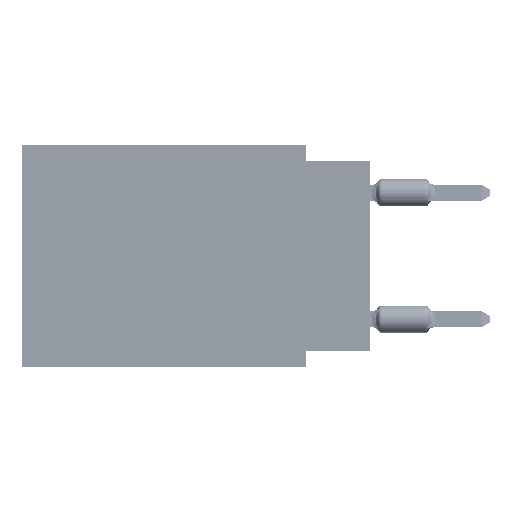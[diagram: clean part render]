
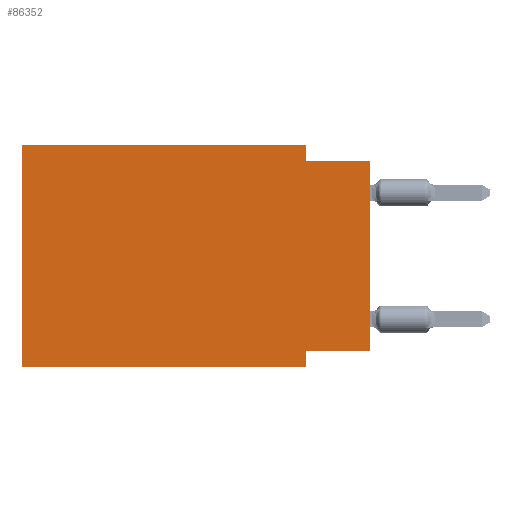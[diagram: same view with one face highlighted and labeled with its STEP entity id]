
A CAD part, left-side view. The second image highlights one B-rep face of the part: STEP entity #86352.
In plain terms, the highlighted planar face has unit normal (-1, 0, 0).
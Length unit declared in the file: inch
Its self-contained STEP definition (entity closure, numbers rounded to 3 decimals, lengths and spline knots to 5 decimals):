
#1003 = ORIENTED_EDGE ( 'NONE', *, *, #39772, .F. ) ;
#2093 = DIRECTION ( 'NONE',  ( 0., 0., -1. ) ) ;
#5446 = DIRECTION ( 'NONE',  ( 0., -1., 0. ) ) ;
#8709 = CARTESIAN_POINT ( 'NONE',  ( 0., 0.1, 0. ) ) ;
#10148 = LINE ( 'NONE', #18905, #48730 ) ;
#13813 = CARTESIAN_POINT ( 'NONE',  ( 0., 0.55, -0.35 ) ) ;
#14261 = LINE ( 'NONE', #49789, #84240 ) ;
#15055 = LINE ( 'NONE', #48445, #47356 ) ;
#15538 = EDGE_CURVE ( 'NONE', #74234, #21049, #10148, .T. ) ;
#16152 = EDGE_CURVE ( 'NONE', #72362, #93234, #98389, .T. ) ;
#17531 = FACE_OUTER_BOUND ( 'NONE', #35085, .T. ) ;
#18905 = CARTESIAN_POINT ( 'NONE',  ( 0., 0., -0.025 ) ) ;
#20301 = VERTEX_POINT ( 'NONE', #31533 ) ;
#21049 = VERTEX_POINT ( 'NONE', #102952 ) ;
#22380 = AXIS2_PLACEMENT_3D ( 'NONE', #33429, #59609, #49814 ) ;
#22952 = CARTESIAN_POINT ( 'NONE',  ( 0., 0.1, -0.325 ) ) ;
#26205 = LINE ( 'NONE', #8709, #44243 ) ;
#26904 = EDGE_CURVE ( 'NONE', #20301, #49916, #27054, .T. ) ;
#27054 = LINE ( 'NONE', #43473, #54297 ) ;
#27501 = ORIENTED_EDGE ( 'NONE', *, *, #15538, .F. ) ;
#27883 = VECTOR ( 'NONE', #5446, 39.37008 ) ;
#27966 = CARTESIAN_POINT ( 'NONE',  ( 0., 0., 0. ) ) ;
#28181 = CARTESIAN_POINT ( 'NONE',  ( 0., 0., -0.325 ) ) ;
#31533 = CARTESIAN_POINT ( 'NONE',  ( 0., 0.55, 0. ) ) ;
#33108 = EDGE_CURVE ( 'NONE', #72362, #20301, #72391, .T. ) ;
#33429 = CARTESIAN_POINT ( 'NONE',  ( 0., 0.55, 0. ) ) ;
#35085 = EDGE_LOOP ( 'NONE', ( #74223, #27501, #106396, #97913, #68588, #54186, #1003, #39846 ) ) ;
#39772 = EDGE_CURVE ( 'NONE', #79829, #93234, #14261, .T. ) ;
#39846 = ORIENTED_EDGE ( 'NONE', *, *, #63535, .F. ) ;
#41630 = PLANE ( 'NONE',  #22380 ) ;
#43473 = CARTESIAN_POINT ( 'NONE',  ( 0., 0.55, 0. ) ) ;
#44243 = VECTOR ( 'NONE', #2093, 39.37008 ) ;
#44535 = VECTOR ( 'NONE', #82196, 39.37008 ) ;
#47356 = VECTOR ( 'NONE', #65923, 39.37008 ) ;
#48445 = CARTESIAN_POINT ( 'NONE',  ( 0., 0., -0.325 ) ) ;
#48730 = VECTOR ( 'NONE', #60441, 39.37008 ) ;
#49789 = CARTESIAN_POINT ( 'NONE',  ( 0., 0.1, -0.35 ) ) ;
#49814 = DIRECTION ( 'NONE',  ( 0., 0., -1. ) ) ;
#49916 = VERTEX_POINT ( 'NONE', #62021 ) ;
#54186 = ORIENTED_EDGE ( 'NONE', *, *, #16152, .T. ) ;
#54297 = VECTOR ( 'NONE', #67006, 39.37008 ) ;
#59609 = DIRECTION ( 'NONE',  ( 1., 0., 0. ) ) ;
#60441 = DIRECTION ( 'NONE',  ( 0., -1., 0. ) ) ;
#62021 = CARTESIAN_POINT ( 'NONE',  ( 0., 0.1, 0. ) ) ;
#63535 = EDGE_CURVE ( 'NONE', #104488, #79829, #15055, .T. ) ;
#65923 = DIRECTION ( 'NONE',  ( 0., 1., 0. ) ) ;
#66745 = DIRECTION ( 'NONE',  ( 0., 0., -1. ) ) ;
#67006 = DIRECTION ( 'NONE',  ( 0., -1., 0. ) ) ;
#68588 = ORIENTED_EDGE ( 'NONE', *, *, #33108, .F. ) ;
#72362 = VERTEX_POINT ( 'NONE', #13813 ) ;
#72391 = LINE ( 'NONE', #90925, #44535 ) ;
#74223 = ORIENTED_EDGE ( 'NONE', *, *, #76300, .T. ) ;
#74234 = VERTEX_POINT ( 'NONE', #105771 ) ;
#76300 = EDGE_CURVE ( 'NONE', #104488, #21049, #103938, .T. ) ;
#79829 = VERTEX_POINT ( 'NONE', #22952 ) ;
#80378 = CARTESIAN_POINT ( 'NONE',  ( 0., 0.55, -0.35 ) ) ;
#82196 = DIRECTION ( 'NONE',  ( 0., 0., 1. ) ) ;
#84240 = VECTOR ( 'NONE', #66745, 39.37008 ) ;
#86352 = ADVANCED_FACE ( 'NONE', ( #17531 ), #41630, .F. ) ;
#90925 = CARTESIAN_POINT ( 'NONE',  ( 0., 0.55, 0. ) ) ;
#92968 = VECTOR ( 'NONE', #94631, 39.37008 ) ;
#93234 = VERTEX_POINT ( 'NONE', #98798 ) ;
#94631 = DIRECTION ( 'NONE',  ( 0., 0., 1. ) ) ;
#95835 = EDGE_CURVE ( 'NONE', #49916, #74234, #26205, .T. ) ;
#97913 = ORIENTED_EDGE ( 'NONE', *, *, #26904, .F. ) ;
#98389 = LINE ( 'NONE', #80378, #27883 ) ;
#98798 = CARTESIAN_POINT ( 'NONE',  ( 0., 0.1, -0.35 ) ) ;
#102952 = CARTESIAN_POINT ( 'NONE',  ( 0., 0., -0.025 ) ) ;
#103938 = LINE ( 'NONE', #27966, #92968 ) ;
#104488 = VERTEX_POINT ( 'NONE', #28181 ) ;
#105771 = CARTESIAN_POINT ( 'NONE',  ( 0., 0.1, -0.025 ) ) ;
#106396 = ORIENTED_EDGE ( 'NONE', *, *, #95835, .F. ) ;
